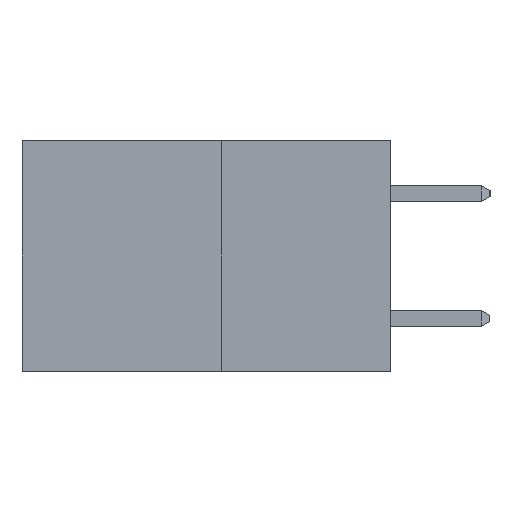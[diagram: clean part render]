
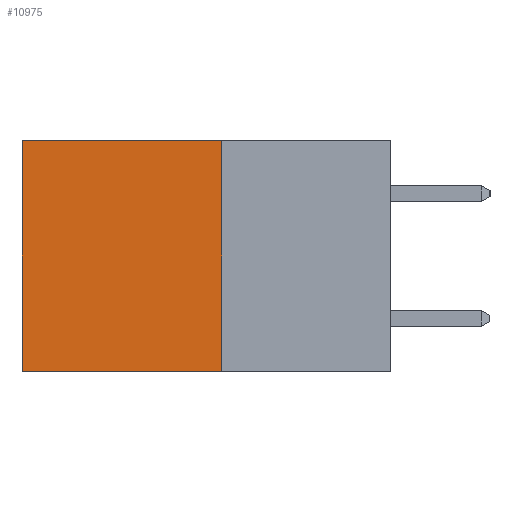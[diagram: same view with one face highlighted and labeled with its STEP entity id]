
A CAD part, left-side view. The second image highlights one B-rep face of the part: STEP entity #10975.
In plain terms, the highlighted planar face has unit normal (-1, 0, 0).
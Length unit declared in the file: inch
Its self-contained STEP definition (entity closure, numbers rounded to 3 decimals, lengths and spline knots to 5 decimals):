
#153 = EDGE_CURVE ( 'NONE', #7833, #9719, #9805, .T. ) ;
#503 = DIRECTION ( 'NONE',  ( 0., 1., 0. ) ) ;
#737 = LINE ( 'NONE', #13811, #12383 ) ;
#1146 = LINE ( 'NONE', #2785, #3769 ) ;
#1338 = CARTESIAN_POINT ( 'NONE',  ( 0.277, 0.59, 0. ) ) ;
#1637 = CARTESIAN_POINT ( 'NONE',  ( 0.277, 0.27, -0.37 ) ) ;
#1764 = VECTOR ( 'NONE', #1946, 39.37008 ) ;
#1938 = ORIENTED_EDGE ( 'NONE', *, *, #7808, .F. ) ;
#1946 = DIRECTION ( 'NONE',  ( 0., 0., -1. ) ) ;
#2785 = CARTESIAN_POINT ( 'NONE',  ( 0.277, 0.27, -0.37 ) ) ;
#3037 = CARTESIAN_POINT ( 'NONE',  ( 0.277, 0.59, -0.37 ) ) ;
#3256 = VERTEX_POINT ( 'NONE', #3037 ) ;
#3363 = EDGE_CURVE ( 'NONE', #7833, #10823, #5150, .T. ) ;
#3769 = VECTOR ( 'NONE', #503, 39.37008 ) ;
#4136 = AXIS2_PLACEMENT_3D ( 'NONE', #9856, #13069, #6644 ) ;
#4632 = EDGE_CURVE ( 'NONE', #9719, #3256, #737, .T. ) ;
#5137 = CARTESIAN_POINT ( 'NONE',  ( 0.277, 0.27, 0. ) ) ;
#5150 = LINE ( 'NONE', #6348, #1764 ) ;
#6186 = ORIENTED_EDGE ( 'NONE', *, *, #153, .T. ) ;
#6348 = CARTESIAN_POINT ( 'NONE',  ( 0.277, 0.27, -0.37 ) ) ;
#6644 = DIRECTION ( 'NONE',  ( 0., 0., -1. ) ) ;
#6893 = CARTESIAN_POINT ( 'NONE',  ( 0.277, 0.27, 0. ) ) ;
#7281 = VECTOR ( 'NONE', #13153, 39.37008 ) ;
#7808 = EDGE_CURVE ( 'NONE', #10823, #3256, #1146, .T. ) ;
#7833 = VERTEX_POINT ( 'NONE', #5137 ) ;
#9719 = VERTEX_POINT ( 'NONE', #1338 ) ;
#9805 = LINE ( 'NONE', #6893, #7281 ) ;
#9856 = CARTESIAN_POINT ( 'NONE',  ( 0.277, 0.27, -0.37 ) ) ;
#10261 = ORIENTED_EDGE ( 'NONE', *, *, #3363, .F. ) ;
#10268 = EDGE_LOOP ( 'NONE', ( #13177, #1938, #10261, #6186 ) ) ;
#10823 = VERTEX_POINT ( 'NONE', #1637 ) ;
#10975 = ADVANCED_FACE ( 'NONE', ( #13158 ), #11950, .F. ) ;
#11950 = PLANE ( 'NONE',  #4136 ) ;
#12383 = VECTOR ( 'NONE', #13440, 39.37008 ) ;
#13069 = DIRECTION ( 'NONE',  ( 1., 0., 0. ) ) ;
#13153 = DIRECTION ( 'NONE',  ( 0., 1., 0. ) ) ;
#13158 = FACE_OUTER_BOUND ( 'NONE', #10268, .T. ) ;
#13177 = ORIENTED_EDGE ( 'NONE', *, *, #4632, .T. ) ;
#13440 = DIRECTION ( 'NONE',  ( 0., 0., -1. ) ) ;
#13811 = CARTESIAN_POINT ( 'NONE',  ( 0.277, 0.59, -0.37 ) ) ;
